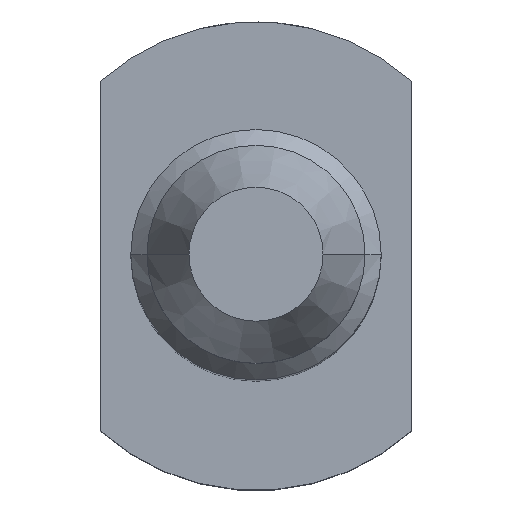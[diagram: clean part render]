
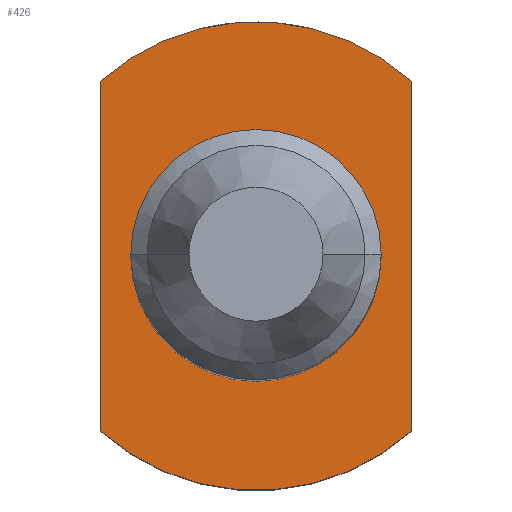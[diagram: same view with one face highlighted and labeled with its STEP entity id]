
A CAD part, top view. The second image highlights one B-rep face of the part: STEP entity #426.
In plain terms, the highlighted planar face has unit normal (0, 0, 1).
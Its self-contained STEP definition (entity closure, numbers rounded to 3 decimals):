
#6 = PLANE ( 'NONE',  #595 ) ;
#13 = CARTESIAN_POINT ( 'NONE',  ( 0.965, 1.082, 0. ) ) ;
#27 = EDGE_CURVE ( 'NONE', #704, #246, #167, .T. ) ;
#30 = CARTESIAN_POINT ( 'NONE',  ( -0.965, -1.082, 0. ) ) ;
#34 = ORIENTED_EDGE ( 'NONE', *, *, #140, .T. ) ;
#59 = DIRECTION ( 'NONE',  ( 0., 1., 0. ) ) ;
#68 = DIRECTION ( 'NONE',  ( 0., 0., -1. ) ) ;
#78 = EDGE_CURVE ( 'NONE', #80, #250, #111, .T. ) ;
#80 = VERTEX_POINT ( 'NONE', #382 ) ;
#99 = FACE_OUTER_BOUND ( 'NONE', #482, .T. ) ;
#111 = LINE ( 'NONE', #502, #156 ) ;
#140 = EDGE_CURVE ( 'NONE', #315, #80, #169, .T. ) ;
#156 = VECTOR ( 'NONE', #59, 1000. ) ;
#167 = CIRCLE ( 'NONE', #489, 0.775 ) ;
#169 = CIRCLE ( 'NONE', #383, 1.45 ) ;
#184 = DIRECTION ( 'NONE',  ( 0., -1., 0. ) ) ;
#196 = CARTESIAN_POINT ( 'NONE',  ( 0., 0., 0. ) ) ;
#226 = DIRECTION ( 'NONE',  ( 0., 0., 1. ) ) ;
#239 = ORIENTED_EDGE ( 'NONE', *, *, #270, .F. ) ;
#243 = CIRCLE ( 'NONE', #445, 0.775 ) ;
#246 = VERTEX_POINT ( 'NONE', #406 ) ;
#250 = VERTEX_POINT ( 'NONE', #13 ) ;
#270 = EDGE_CURVE ( 'NONE', #317, #250, #346, .T. ) ;
#272 = DIRECTION ( 'NONE',  ( -1., 0., 0. ) ) ;
#277 = EDGE_CURVE ( 'NONE', #317, #315, #630, .T. ) ;
#281 = FACE_BOUND ( 'NONE', #310, .T. ) ;
#305 = ORIENTED_EDGE ( 'NONE', *, *, #277, .T. ) ;
#306 = CARTESIAN_POINT ( 'NONE',  ( -0.965, 1.082, 0. ) ) ;
#309 = VECTOR ( 'NONE', #184, 1000. ) ;
#310 = EDGE_LOOP ( 'NONE', ( #671, #686 ) ) ;
#315 = VERTEX_POINT ( 'NONE', #30 ) ;
#317 = VERTEX_POINT ( 'NONE', #306 ) ;
#336 = CARTESIAN_POINT ( 'NONE',  ( 0., 0., 0. ) ) ;
#346 = CIRCLE ( 'NONE', #444, 1.45 ) ;
#368 = DIRECTION ( 'NONE',  ( 0., 0., 1. ) ) ;
#382 = CARTESIAN_POINT ( 'NONE',  ( 0.965, -1.082, 0. ) ) ;
#383 = AXIS2_PLACEMENT_3D ( 'NONE', #449, #562, #694 ) ;
#403 = CARTESIAN_POINT ( 'NONE',  ( -0.965, 1.082, 0. ) ) ;
#406 = CARTESIAN_POINT ( 'NONE',  ( 0.775, 0., 0. ) ) ;
#409 = CARTESIAN_POINT ( 'NONE',  ( 0., 0., 0. ) ) ;
#420 = ORIENTED_EDGE ( 'NONE', *, *, #78, .T. ) ;
#426 = ADVANCED_FACE ( 'NONE', ( #281, #99 ), #6, .T. ) ;
#442 = DIRECTION ( 'NONE',  ( 0., 0., -1. ) ) ;
#444 = AXIS2_PLACEMENT_3D ( 'NONE', #409, #68, #465 ) ;
#445 = AXIS2_PLACEMENT_3D ( 'NONE', #336, #442, #506 ) ;
#449 = CARTESIAN_POINT ( 'NONE',  ( 0., 0., 0. ) ) ;
#461 = CARTESIAN_POINT ( 'NONE',  ( -0.775, 0., 0. ) ) ;
#465 = DIRECTION ( 'NONE',  ( 1., 0., 0. ) ) ;
#482 = EDGE_LOOP ( 'NONE', ( #239, #305, #34, #420 ) ) ;
#489 = AXIS2_PLACEMENT_3D ( 'NONE', #196, #368, #661 ) ;
#502 = CARTESIAN_POINT ( 'NONE',  ( 0.965, -1.082, 0. ) ) ;
#506 = DIRECTION ( 'NONE',  ( -1., 0., 0. ) ) ;
#534 = EDGE_CURVE ( 'NONE', #704, #246, #243, .T. ) ;
#562 = DIRECTION ( 'NONE',  ( 0., 0., 1. ) ) ;
#595 = AXIS2_PLACEMENT_3D ( 'NONE', #667, #226, #272 ) ;
#630 = LINE ( 'NONE', #403, #309 ) ;
#661 = DIRECTION ( 'NONE',  ( -1., 0., 0. ) ) ;
#667 = CARTESIAN_POINT ( 'NONE',  ( 0., 0., 0. ) ) ;
#671 = ORIENTED_EDGE ( 'NONE', *, *, #534, .T. ) ;
#686 = ORIENTED_EDGE ( 'NONE', *, *, #27, .F. ) ;
#694 = DIRECTION ( 'NONE',  ( -0.666, -0.746, 0. ) ) ;
#704 = VERTEX_POINT ( 'NONE', #461 ) ;
